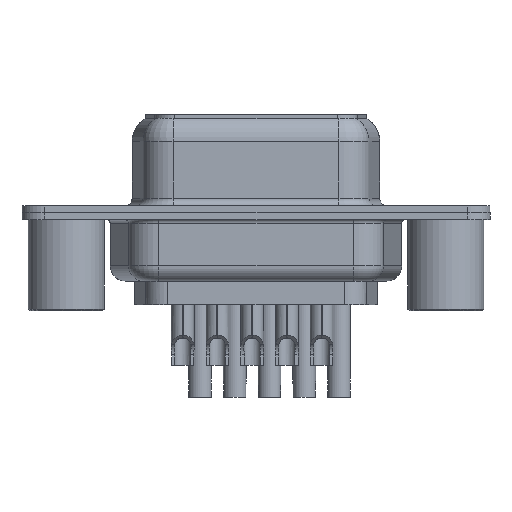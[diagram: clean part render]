
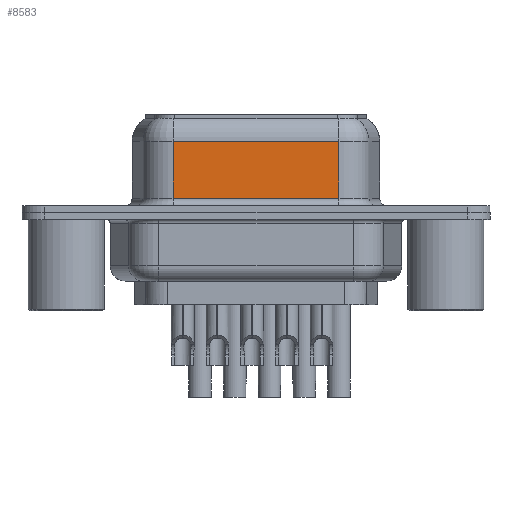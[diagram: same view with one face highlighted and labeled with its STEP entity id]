
A CAD part, front view. The second image highlights one B-rep face of the part: STEP entity #8583.
In plain terms, the highlighted planar face has unit normal (0, -1, 0).
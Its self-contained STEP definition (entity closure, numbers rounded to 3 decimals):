
#351 = LINE ( 'NONE', #4059, #23779 ) ;
#694 = LINE ( 'NONE', #2725, #11270 ) ;
#1392 = VERTEX_POINT ( 'NONE', #12273 ) ;
#2725 = CARTESIAN_POINT ( 'NONE',  ( 17.957, -3.95, 4.7 ) ) ;
#3005 = PLANE ( 'NONE',  #14785 ) ;
#3071 = CARTESIAN_POINT ( 'NONE',  ( 17.957, -3.95, 6.45 ) ) ;
#3199 = DIRECTION ( 'NONE',  ( 0., 0., -1. ) ) ;
#3518 = FACE_OUTER_BOUND ( 'NONE', #19156, .T. ) ;
#4059 = CARTESIAN_POINT ( 'NONE',  ( 17.957, -3.95, 0.95 ) ) ;
#4333 = VERTEX_POINT ( 'NONE', #4723 ) ;
#4723 = CARTESIAN_POINT ( 'NONE',  ( 7.033, -3.95, 0.95 ) ) ;
#6267 = EDGE_CURVE ( 'NONE', #21042, #6693, #694, .T. ) ;
#6693 = VERTEX_POINT ( 'NONE', #7458 ) ;
#7125 = DIRECTION ( 'NONE',  ( 0., 1., 0. ) ) ;
#7458 = CARTESIAN_POINT ( 'NONE',  ( 7.033, -3.95, 4.7 ) ) ;
#7952 = CARTESIAN_POINT ( 'NONE',  ( 7.033, -3.95, 6.45 ) ) ;
#8583 = ADVANCED_FACE ( 'NONE', ( #3518 ), #3005, .F. ) ;
#8921 = DIRECTION ( 'NONE',  ( -1., 0., 0. ) ) ;
#11270 = VECTOR ( 'NONE', #8921, 1000. ) ;
#11371 = LINE ( 'NONE', #7952, #12397 ) ;
#11653 = EDGE_CURVE ( 'NONE', #4333, #1392, #351, .T. ) ;
#11863 = DIRECTION ( 'NONE',  ( 1., 0., 0. ) ) ;
#12273 = CARTESIAN_POINT ( 'NONE',  ( 17.957, -3.95, 0.95 ) ) ;
#12397 = VECTOR ( 'NONE', #21336, 1000. ) ;
#12507 = EDGE_CURVE ( 'NONE', #6693, #4333, #11371, .T. ) ;
#12899 = VECTOR ( 'NONE', #3199, 1000. ) ;
#14785 = AXIS2_PLACEMENT_3D ( 'NONE', #19088, #7125, #15150 ) ;
#15150 = DIRECTION ( 'NONE',  ( 0., 0., 1. ) ) ;
#16616 = LINE ( 'NONE', #3071, #12899 ) ;
#16728 = EDGE_CURVE ( 'NONE', #21042, #1392, #16616, .T. ) ;
#19088 = CARTESIAN_POINT ( 'NONE',  ( 17.957, -3.95, 6.45 ) ) ;
#19156 = EDGE_LOOP ( 'NONE', ( #20741, #25144, #22693, #19292 ) ) ;
#19292 = ORIENTED_EDGE ( 'NONE', *, *, #11653, .T. ) ;
#20741 = ORIENTED_EDGE ( 'NONE', *, *, #16728, .F. ) ;
#21042 = VERTEX_POINT ( 'NONE', #22466 ) ;
#21336 = DIRECTION ( 'NONE',  ( 0., 0., -1. ) ) ;
#22466 = CARTESIAN_POINT ( 'NONE',  ( 17.957, -3.95, 4.7 ) ) ;
#22693 = ORIENTED_EDGE ( 'NONE', *, *, #12507, .T. ) ;
#23779 = VECTOR ( 'NONE', #11863, 1000. ) ;
#25144 = ORIENTED_EDGE ( 'NONE', *, *, #6267, .T. ) ;
